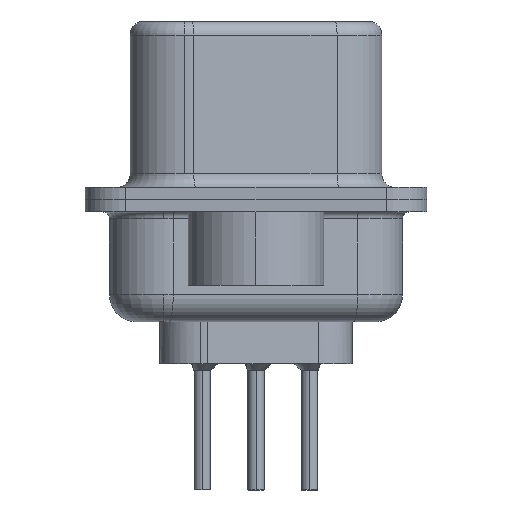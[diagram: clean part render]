
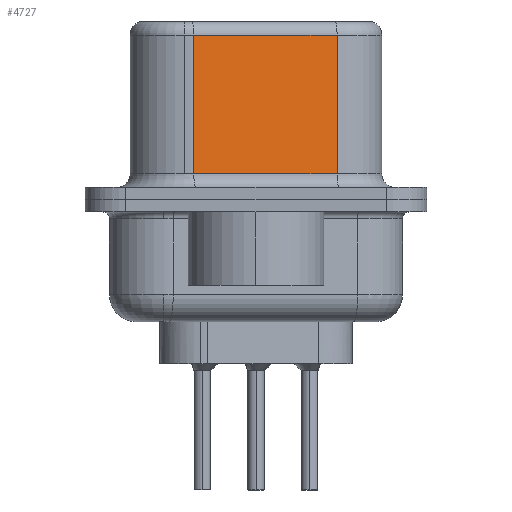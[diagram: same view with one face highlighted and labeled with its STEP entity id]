
A CAD part, left-side view. The second image highlights one B-rep face of the part: STEP entity #4727.
In plain terms, the highlighted planar face has unit normal (-0.985, -0.174, 0).
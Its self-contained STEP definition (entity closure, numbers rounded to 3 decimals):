
#254 = PLANE ( 'NONE',  #4620 ) ;
#1939 = CARTESIAN_POINT ( 'NONE',  ( 3.615, 2.293, 6.07 ) ) ;
#2173 = CARTESIAN_POINT ( 'NONE',  ( 3.615, 2.293, 6.57 ) ) ;
#2821 = LINE ( 'NONE', #4325, #3096 ) ;
#3019 = LINE ( 'NONE', #3260, #16868 ) ;
#3096 = VECTOR ( 'NONE', #12501, 1000. ) ;
#3260 = CARTESIAN_POINT ( 'NONE',  ( 4.546, -2.987, 0.95 ) ) ;
#3767 = VERTEX_POINT ( 'NONE', #4996 ) ;
#4325 = CARTESIAN_POINT ( 'NONE',  ( 4.546, -2.987, 6.07 ) ) ;
#4620 = AXIS2_PLACEMENT_3D ( 'NONE', #9257, #21985, #11152 ) ;
#4727 = ADVANCED_FACE ( 'NONE', ( #18771 ), #254, .F. ) ;
#4996 = CARTESIAN_POINT ( 'NONE',  ( 3.615, 2.293, 0.95 ) ) ;
#5974 = VECTOR ( 'NONE', #22026, 1000. ) ;
#6998 = EDGE_CURVE ( 'NONE', #8839, #3767, #10232, .T. ) ;
#7688 = ORIENTED_EDGE ( 'NONE', *, *, #22373, .T. ) ;
#8257 = ORIENTED_EDGE ( 'NONE', *, *, #16009, .T. ) ;
#8659 = DIRECTION ( 'NONE',  ( 0.174, -0.985, 0. ) ) ;
#8839 = VERTEX_POINT ( 'NONE', #1939 ) ;
#9127 = VECTOR ( 'NONE', #18274, 1000. ) ;
#9257 = CARTESIAN_POINT ( 'NONE',  ( 4.546, -2.987, 6.57 ) ) ;
#10232 = LINE ( 'NONE', #2173, #5974 ) ;
#10454 = CARTESIAN_POINT ( 'NONE',  ( 4.546, -2.987, 6.07 ) ) ;
#10963 = CARTESIAN_POINT ( 'NONE',  ( 4.546, -2.987, 6.57 ) ) ;
#11152 = DIRECTION ( 'NONE',  ( -0.174, 0.985, 0. ) ) ;
#12501 = DIRECTION ( 'NONE',  ( -0.174, 0.985, 0. ) ) ;
#13921 = LINE ( 'NONE', #10963, #9127 ) ;
#14973 = VERTEX_POINT ( 'NONE', #10454 ) ;
#16009 = EDGE_CURVE ( 'NONE', #3767, #21496, #3019, .T. ) ;
#16124 = CARTESIAN_POINT ( 'NONE',  ( 4.546, -2.987, 0.95 ) ) ;
#16868 = VECTOR ( 'NONE', #8659, 1000. ) ;
#18010 = ORIENTED_EDGE ( 'NONE', *, *, #21305, .F. ) ;
#18046 = EDGE_LOOP ( 'NONE', ( #18010, #7688, #20740, #8257 ) ) ;
#18274 = DIRECTION ( 'NONE',  ( 0., 0., -1. ) ) ;
#18771 = FACE_OUTER_BOUND ( 'NONE', #18046, .T. ) ;
#20740 = ORIENTED_EDGE ( 'NONE', *, *, #6998, .T. ) ;
#21305 = EDGE_CURVE ( 'NONE', #14973, #21496, #13921, .T. ) ;
#21496 = VERTEX_POINT ( 'NONE', #16124 ) ;
#21985 = DIRECTION ( 'NONE',  ( 0.985, 0.174, 0. ) ) ;
#22026 = DIRECTION ( 'NONE',  ( 0., 0., -1. ) ) ;
#22373 = EDGE_CURVE ( 'NONE', #14973, #8839, #2821, .T. ) ;
